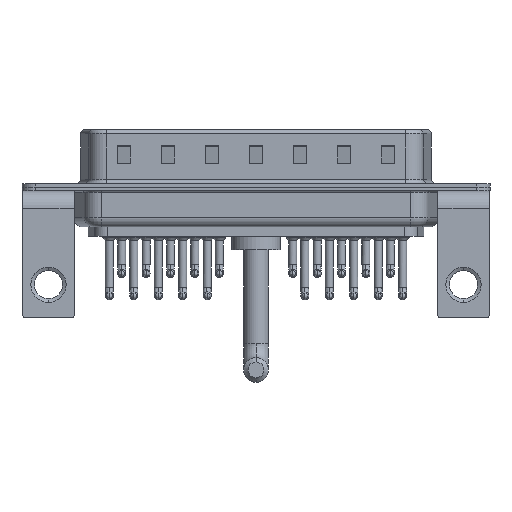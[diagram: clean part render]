
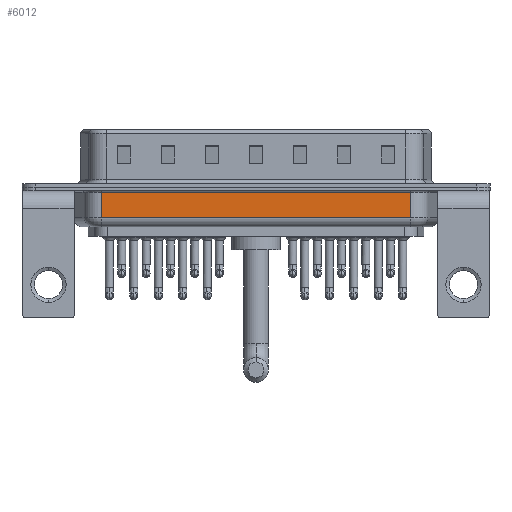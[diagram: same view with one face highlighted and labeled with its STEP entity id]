
A CAD part, front view. The second image highlights one B-rep face of the part: STEP entity #6012.
In plain terms, the highlighted planar face has unit normal (0, -1, 0).
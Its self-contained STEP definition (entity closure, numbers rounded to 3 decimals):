
#971 = FACE_OUTER_BOUND ( 'NONE', #18433, .T. ) ;
#2107 = LINE ( 'NONE', #14781, #17543 ) ;
#2296 = VERTEX_POINT ( 'NONE', #26569 ) ;
#2446 = CARTESIAN_POINT ( 'NONE',  ( 41.044, -5.35, -0.65 ) ) ;
#2717 = EDGE_CURVE ( 'NONE', #17641, #26645, #2107, .T. ) ;
#2887 = DIRECTION ( 'NONE',  ( 0., 1., 0. ) ) ;
#3134 = PLANE ( 'NONE',  #13374 ) ;
#3285 = LINE ( 'NONE', #7594, #25578 ) ;
#4153 = ORIENTED_EDGE ( 'NONE', *, *, #9509, .T. ) ;
#4339 = CARTESIAN_POINT ( 'NONE',  ( 6.006, -5.35, -4.5 ) ) ;
#5350 = DIRECTION ( 'NONE',  ( -1., 0., 0. ) ) ;
#6012 = ADVANCED_FACE ( 'NONE', ( #971 ), #3134, .F. ) ;
#6922 = CARTESIAN_POINT ( 'NONE',  ( 6.006, -5.35, -3.5 ) ) ;
#7361 = VERTEX_POINT ( 'NONE', #6922 ) ;
#7594 = CARTESIAN_POINT ( 'NONE',  ( 6.006, -5.35, -3.5 ) ) ;
#8255 = ORIENTED_EDGE ( 'NONE', *, *, #14267, .T. ) ;
#8375 = LINE ( 'NONE', #4339, #26502 ) ;
#8530 = DIRECTION ( 'NONE',  ( 0., 0., 1. ) ) ;
#8964 = CARTESIAN_POINT ( 'NONE',  ( 6.006, -5.35, -4.5 ) ) ;
#9142 = CARTESIAN_POINT ( 'NONE',  ( 6.006, -5.35, -0.65 ) ) ;
#9509 = EDGE_CURVE ( 'NONE', #7361, #17641, #3285, .T. ) ;
#12962 = ORIENTED_EDGE ( 'NONE', *, *, #26607, .F. ) ;
#13374 = AXIS2_PLACEMENT_3D ( 'NONE', #8964, #2887, #19325 ) ;
#14267 = EDGE_CURVE ( 'NONE', #26645, #2296, #21539, .T. ) ;
#14781 = CARTESIAN_POINT ( 'NONE',  ( 41.044, -5.35, -4.5 ) ) ;
#17543 = VECTOR ( 'NONE', #26495, 1000. ) ;
#17641 = VERTEX_POINT ( 'NONE', #17961 ) ;
#17961 = CARTESIAN_POINT ( 'NONE',  ( 41.044, -5.35, -3.5 ) ) ;
#18433 = EDGE_LOOP ( 'NONE', ( #12962, #4153, #25925, #8255 ) ) ;
#19325 = DIRECTION ( 'NONE',  ( 0., 0., 1. ) ) ;
#19740 = DIRECTION ( 'NONE',  ( 1., 0., 0. ) ) ;
#21539 = LINE ( 'NONE', #9142, #24678 ) ;
#24678 = VECTOR ( 'NONE', #5350, 1000. ) ;
#25578 = VECTOR ( 'NONE', #19740, 1000. ) ;
#25925 = ORIENTED_EDGE ( 'NONE', *, *, #2717, .T. ) ;
#26495 = DIRECTION ( 'NONE',  ( 0., 0., 1. ) ) ;
#26502 = VECTOR ( 'NONE', #8530, 1000. ) ;
#26569 = CARTESIAN_POINT ( 'NONE',  ( 6.006, -5.35, -0.65 ) ) ;
#26607 = EDGE_CURVE ( 'NONE', #7361, #2296, #8375, .T. ) ;
#26645 = VERTEX_POINT ( 'NONE', #2446 ) ;
